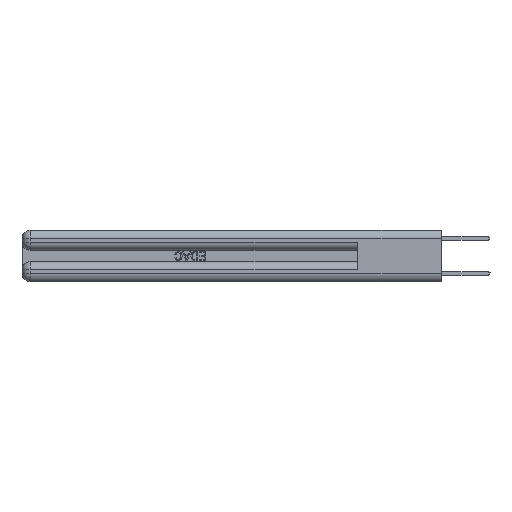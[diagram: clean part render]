
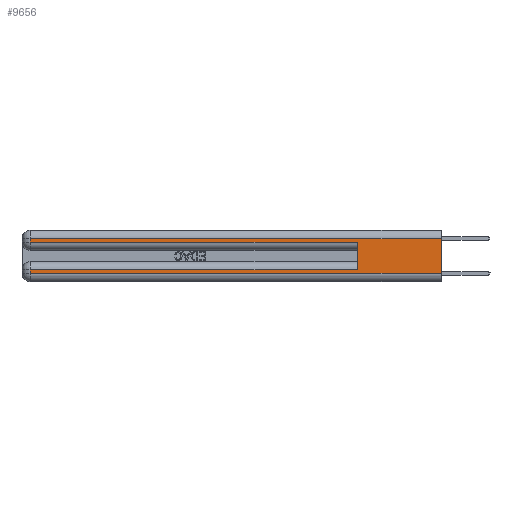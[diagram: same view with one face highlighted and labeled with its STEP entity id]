
A CAD part, left-side view. The second image highlights one B-rep face of the part: STEP entity #9656.
In plain terms, the highlighted planar face has unit normal (-1, 0, 0).
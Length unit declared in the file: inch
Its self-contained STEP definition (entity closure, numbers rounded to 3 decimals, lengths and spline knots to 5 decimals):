
#342 = DIRECTION ( 'NONE',  ( 1., 0., 0. ) ) ;
#496 = CARTESIAN_POINT ( 'NONE',  ( 0., 0., 0.285 ) ) ;
#626 = VERTEX_POINT ( 'NONE', #20506 ) ;
#2193 = LINE ( 'NONE', #29823, #27422 ) ;
#2518 = CARTESIAN_POINT ( 'NONE',  ( 0., 0., 0.06 ) ) ;
#3063 = DIRECTION ( 'NONE',  ( 0., -1., 0. ) ) ;
#3133 = PLANE ( 'NONE',  #27496 ) ;
#3170 = DIRECTION ( 'NONE',  ( 0., 1., 0. ) ) ;
#3730 = CARTESIAN_POINT ( 'NONE',  ( 0., 2.94, 0.37 ) ) ;
#4045 = VERTEX_POINT ( 'NONE', #4748 ) ;
#4335 = DIRECTION ( 'NONE',  ( 0., 1., 0. ) ) ;
#4748 = CARTESIAN_POINT ( 'NONE',  ( 0., 0.6, 0.085 ) ) ;
#5226 = LINE ( 'NONE', #20280, #29257 ) ;
#5334 = LINE ( 'NONE', #496, #8871 ) ;
#5466 = LINE ( 'NONE', #17919, #12938 ) ;
#5552 = CARTESIAN_POINT ( 'NONE',  ( 0., 2.94, 0.31 ) ) ;
#6267 = DIRECTION ( 'NONE',  ( 0., 0., -1. ) ) ;
#7718 = EDGE_CURVE ( 'NONE', #21680, #8650, #5226, .T. ) ;
#7891 = ORIENTED_EDGE ( 'NONE', *, *, #25941, .T. ) ;
#8650 = VERTEX_POINT ( 'NONE', #2518 ) ;
#8871 = VECTOR ( 'NONE', #3063, 39.37008 ) ;
#8934 = VERTEX_POINT ( 'NONE', #21310 ) ;
#9656 = ADVANCED_FACE ( 'NONE', ( #29883 ), #3133, .F. ) ;
#9850 = ORIENTED_EDGE ( 'NONE', *, *, #11423, .T. ) ;
#9952 = DIRECTION ( 'NONE',  ( 0., 0., 1. ) ) ;
#11423 = EDGE_CURVE ( 'NONE', #8934, #626, #18253, .T. ) ;
#12015 = ORIENTED_EDGE ( 'NONE', *, *, #23434, .T. ) ;
#12225 = ORIENTED_EDGE ( 'NONE', *, *, #16698, .T. ) ;
#12245 = LINE ( 'NONE', #17190, #27226 ) ;
#12261 = CARTESIAN_POINT ( 'NONE',  ( 0., 0.6, 0.145 ) ) ;
#12938 = VECTOR ( 'NONE', #3170, 39.37008 ) ;
#13055 = CARTESIAN_POINT ( 'NONE',  ( 0., 0., 0.06 ) ) ;
#13341 = ORIENTED_EDGE ( 'NONE', *, *, #24005, .F. ) ;
#13924 = VECTOR ( 'NONE', #6267, 39.37008 ) ;
#14342 = EDGE_LOOP ( 'NONE', ( #20716, #22584, #7891, #12225, #13341, #19883, #9850, #12015 ) ) ;
#15047 = EDGE_CURVE ( 'NONE', #21680, #30327, #5466, .T. ) ;
#15070 = CARTESIAN_POINT ( 'NONE',  ( 0., 2.94, 0.285 ) ) ;
#16698 = EDGE_CURVE ( 'NONE', #18468, #31962, #5334, .T. ) ;
#17190 = CARTESIAN_POINT ( 'NONE',  ( 0., 0., 0.085 ) ) ;
#17919 = CARTESIAN_POINT ( 'NONE',  ( 0., 0., 0.31 ) ) ;
#18253 = LINE ( 'NONE', #3730, #13924 ) ;
#18468 = VERTEX_POINT ( 'NONE', #15070 ) ;
#19082 = LINE ( 'NONE', #13055, #24981 ) ;
#19475 = EDGE_CURVE ( 'NONE', #4045, #8934, #12245, .T. ) ;
#19883 = ORIENTED_EDGE ( 'NONE', *, *, #19475, .T. ) ;
#20280 = CARTESIAN_POINT ( 'NONE',  ( 0., 0., 0.37 ) ) ;
#20506 = CARTESIAN_POINT ( 'NONE',  ( 0., 2.94, 0.06 ) ) ;
#20612 = CARTESIAN_POINT ( 'NONE',  ( 0., 0., 0.37 ) ) ;
#20634 = DIRECTION ( 'NONE',  ( 0., -1., 0. ) ) ;
#20716 = ORIENTED_EDGE ( 'NONE', *, *, #7718, .F. ) ;
#21220 = CARTESIAN_POINT ( 'NONE',  ( 0., 0., 0.31 ) ) ;
#21310 = CARTESIAN_POINT ( 'NONE',  ( 0., 2.94, 0.085 ) ) ;
#21680 = VERTEX_POINT ( 'NONE', #21220 ) ;
#22584 = ORIENTED_EDGE ( 'NONE', *, *, #15047, .T. ) ;
#23434 = EDGE_CURVE ( 'NONE', #626, #8650, #19082, .T. ) ;
#24005 = EDGE_CURVE ( 'NONE', #4045, #31962, #30641, .T. ) ;
#24210 = CARTESIAN_POINT ( 'NONE',  ( 0., 0.6, 0.285 ) ) ;
#24981 = VECTOR ( 'NONE', #20634, 39.37008 ) ;
#25941 = EDGE_CURVE ( 'NONE', #30327, #18468, #2193, .T. ) ;
#27226 = VECTOR ( 'NONE', #4335, 39.37008 ) ;
#27422 = VECTOR ( 'NONE', #32576, 39.37008 ) ;
#27496 = AXIS2_PLACEMENT_3D ( 'NONE', #20612, #342, #30855 ) ;
#27900 = DIRECTION ( 'NONE',  ( 0., 0., -1. ) ) ;
#29257 = VECTOR ( 'NONE', #27900, 39.37008 ) ;
#29823 = CARTESIAN_POINT ( 'NONE',  ( 0., 2.94, 0.37 ) ) ;
#29883 = FACE_OUTER_BOUND ( 'NONE', #14342, .T. ) ;
#30265 = VECTOR ( 'NONE', #9952, 39.37008 ) ;
#30327 = VERTEX_POINT ( 'NONE', #5552 ) ;
#30641 = LINE ( 'NONE', #12261, #30265 ) ;
#30855 = DIRECTION ( 'NONE',  ( 0., 0., -1. ) ) ;
#31962 = VERTEX_POINT ( 'NONE', #24210 ) ;
#32576 = DIRECTION ( 'NONE',  ( 0., 0., -1. ) ) ;
